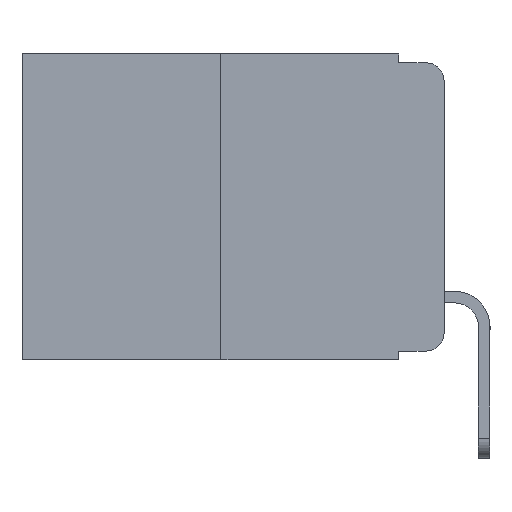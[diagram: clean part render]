
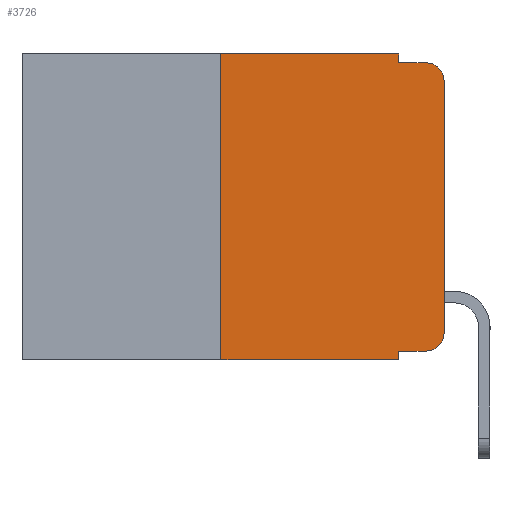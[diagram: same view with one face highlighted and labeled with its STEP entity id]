
A CAD part, left-side view. The second image highlights one B-rep face of the part: STEP entity #3726.
In plain terms, the highlighted planar face has unit normal (-1, 0, 0).
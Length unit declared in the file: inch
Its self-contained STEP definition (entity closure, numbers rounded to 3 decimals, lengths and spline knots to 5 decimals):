
#14 = VERTEX_POINT ( 'NONE', #675 ) ;
#34 = VERTEX_POINT ( 'NONE', #9338 ) ;
#176 = DIRECTION ( 'NONE',  ( 0., -1., 0. ) ) ;
#222 = EDGE_CURVE ( 'NONE', #14, #34, #10322, .T. ) ;
#423 = EDGE_CURVE ( 'NONE', #7598, #793, #6201, .T. ) ;
#525 = EDGE_CURVE ( 'NONE', #2851, #3629, #11672, .T. ) ;
#675 = CARTESIAN_POINT ( 'NONE',  ( 0., 0.051, -0.01 ) ) ;
#723 = CARTESIAN_POINT ( 'NONE',  ( 0., 0.051, 0. ) ) ;
#772 = AXIS2_PLACEMENT_3D ( 'NONE', #10731, #7976, #8859 ) ;
#793 = VERTEX_POINT ( 'NONE', #12283 ) ;
#1107 = LINE ( 'NONE', #11337, #3561 ) ;
#1203 = ORIENTED_EDGE ( 'NONE', *, *, #6744, .T. ) ;
#1561 = ORIENTED_EDGE ( 'NONE', *, *, #10217, .F. ) ;
#1735 = ORIENTED_EDGE ( 'NONE', *, *, #10733, .F. ) ;
#1748 = ORIENTED_EDGE ( 'NONE', *, *, #4072, .F. ) ;
#1780 = LINE ( 'NONE', #5332, #6713 ) ;
#1902 = ORIENTED_EDGE ( 'NONE', *, *, #11711, .T. ) ;
#1917 = DIRECTION ( 'NONE',  ( 0., 0., -1. ) ) ;
#2081 = ORIENTED_EDGE ( 'NONE', *, *, #525, .F. ) ;
#2083 = VERTEX_POINT ( 'NONE', #10425 ) ;
#2247 = CARTESIAN_POINT ( 'NONE',  ( 0., 0., -0.313 ) ) ;
#2310 = AXIS2_PLACEMENT_3D ( 'NONE', #9775, #4244, #10640 ) ;
#2494 = ORIENTED_EDGE ( 'NONE', *, *, #5567, .T. ) ;
#2631 = DIRECTION ( 'NONE',  ( 0., 0., -1. ) ) ;
#2851 = VERTEX_POINT ( 'NONE', #7850 ) ;
#2882 = LINE ( 'NONE', #3585, #5220 ) ;
#2927 = EDGE_CURVE ( 'NONE', #5636, #7598, #11422, .T. ) ;
#3014 = VECTOR ( 'NONE', #11050, 39.37008 ) ;
#3494 = CARTESIAN_POINT ( 'NONE',  ( 0., 0.02, -0.333 ) ) ;
#3561 = VECTOR ( 'NONE', #11949, 39.37008 ) ;
#3585 = CARTESIAN_POINT ( 'NONE',  ( 0., 0.473, 0. ) ) ;
#3629 = VERTEX_POINT ( 'NONE', #4186 ) ;
#3679 = ORIENTED_EDGE ( 'NONE', *, *, #2927, .T. ) ;
#3726 = ADVANCED_FACE ( 'NONE', ( #12348 ), #11400, .F. ) ;
#3998 = DIRECTION ( 'NONE',  ( 0., -1., 0. ) ) ;
#4072 = EDGE_CURVE ( 'NONE', #9471, #2083, #8777, .T. ) ;
#4186 = CARTESIAN_POINT ( 'NONE',  ( 0., 0.051, -0.343 ) ) ;
#4244 = DIRECTION ( 'NONE',  ( -1., 0., 0. ) ) ;
#4582 = DIRECTION ( 'NONE',  ( 0., -1., 0. ) ) ;
#4934 = CARTESIAN_POINT ( 'NONE',  ( 0., 0., 0. ) ) ;
#4951 = CARTESIAN_POINT ( 'NONE',  ( 0., 0.051, 0. ) ) ;
#5220 = VECTOR ( 'NONE', #4582, 39.37008 ) ;
#5231 = VECTOR ( 'NONE', #1917, 39.37008 ) ;
#5332 = CARTESIAN_POINT ( 'NONE',  ( 0., 0.051, -0.333 ) ) ;
#5567 = EDGE_CURVE ( 'NONE', #2851, #5636, #1780, .T. ) ;
#5636 = VERTEX_POINT ( 'NONE', #3494 ) ;
#6201 = LINE ( 'NONE', #4934, #3014 ) ;
#6713 = VECTOR ( 'NONE', #176, 39.37008 ) ;
#6744 = EDGE_CURVE ( 'NONE', #793, #34, #7845, .T. ) ;
#6949 = AXIS2_PLACEMENT_3D ( 'NONE', #7952, #7949, #8029 ) ;
#7598 = VERTEX_POINT ( 'NONE', #2247 ) ;
#7712 = LINE ( 'NONE', #4951, #5231 ) ;
#7845 = CIRCLE ( 'NONE', #2310, 0.02 ) ;
#7850 = CARTESIAN_POINT ( 'NONE',  ( 0., 0.051, -0.333 ) ) ;
#7866 = CARTESIAN_POINT ( 'NONE',  ( 0., 0.25, -0.343 ) ) ;
#7949 = DIRECTION ( 'NONE',  ( -1., 0., 0. ) ) ;
#7952 = CARTESIAN_POINT ( 'NONE',  ( 0., 0.02, -0.313 ) ) ;
#7976 = DIRECTION ( 'NONE',  ( 1., 0., 0. ) ) ;
#8001 = DIRECTION ( 'NONE',  ( 0., 0., 1. ) ) ;
#8029 = DIRECTION ( 'NONE',  ( 0., 0., -1. ) ) ;
#8777 = LINE ( 'NONE', #9816, #10829 ) ;
#8859 = DIRECTION ( 'NONE',  ( 0., 0., -1. ) ) ;
#9338 = CARTESIAN_POINT ( 'NONE',  ( 0., 0.02, -0.01 ) ) ;
#9350 = VECTOR ( 'NONE', #2631, 39.37008 ) ;
#9471 = VERTEX_POINT ( 'NONE', #7866 ) ;
#9775 = CARTESIAN_POINT ( 'NONE',  ( 0., 0.02, -0.03 ) ) ;
#9816 = CARTESIAN_POINT ( 'NONE',  ( 0., 0.25, 0. ) ) ;
#10042 = VECTOR ( 'NONE', #3998, 39.37008 ) ;
#10217 = EDGE_CURVE ( 'NONE', #11074, #14, #7712, .T. ) ;
#10322 = LINE ( 'NONE', #10675, #10042 ) ;
#10425 = CARTESIAN_POINT ( 'NONE',  ( 0., 0.25, 0. ) ) ;
#10640 = DIRECTION ( 'NONE',  ( 0., 0., -1. ) ) ;
#10675 = CARTESIAN_POINT ( 'NONE',  ( 0., 0.051, -0.01 ) ) ;
#10731 = CARTESIAN_POINT ( 'NONE',  ( 0., 0.473, 0. ) ) ;
#10733 = EDGE_CURVE ( 'NONE', #2083, #11074, #2882, .T. ) ;
#10829 = VECTOR ( 'NONE', #8001, 39.37008 ) ;
#10850 = EDGE_LOOP ( 'NONE', ( #10978, #1203, #12086, #1561, #1735, #1748, #1902, #2081, #2494, #3679 ) ) ;
#10978 = ORIENTED_EDGE ( 'NONE', *, *, #423, .T. ) ;
#11050 = DIRECTION ( 'NONE',  ( 0., 0., 1. ) ) ;
#11074 = VERTEX_POINT ( 'NONE', #11485 ) ;
#11337 = CARTESIAN_POINT ( 'NONE',  ( 0., 0.473, -0.343 ) ) ;
#11400 = PLANE ( 'NONE',  #772 ) ;
#11422 = CIRCLE ( 'NONE', #6949, 0.02 ) ;
#11485 = CARTESIAN_POINT ( 'NONE',  ( 0., 0.051, 0. ) ) ;
#11672 = LINE ( 'NONE', #723, #9350 ) ;
#11711 = EDGE_CURVE ( 'NONE', #9471, #3629, #1107, .T. ) ;
#11949 = DIRECTION ( 'NONE',  ( 0., -1., 0. ) ) ;
#12086 = ORIENTED_EDGE ( 'NONE', *, *, #222, .F. ) ;
#12283 = CARTESIAN_POINT ( 'NONE',  ( 0., 0., -0.03 ) ) ;
#12348 = FACE_OUTER_BOUND ( 'NONE', #10850, .T. ) ;
